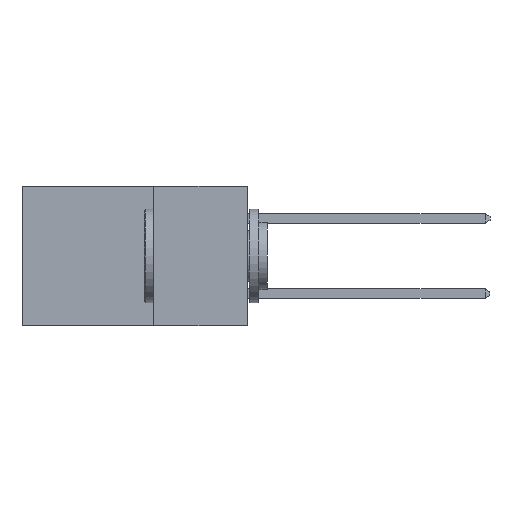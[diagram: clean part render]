
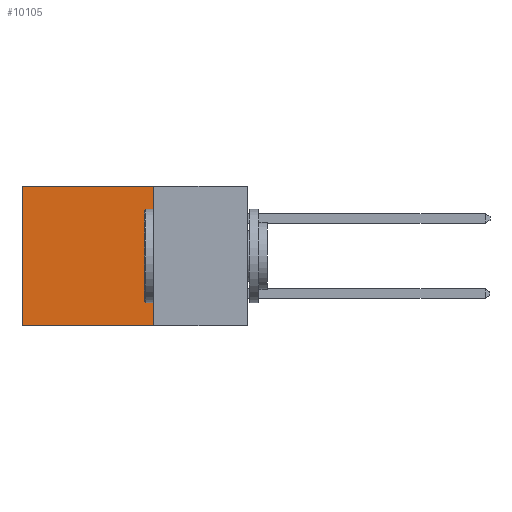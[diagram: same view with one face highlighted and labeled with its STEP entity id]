
A CAD part, left-side view. The second image highlights one B-rep face of the part: STEP entity #10105.
In plain terms, the highlighted planar face has unit normal (-1, 0, 0).
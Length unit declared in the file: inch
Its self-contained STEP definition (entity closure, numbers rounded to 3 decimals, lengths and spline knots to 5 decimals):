
#610 = LINE ( 'NONE', #11379, #5874 ) ;
#1391 = CARTESIAN_POINT ( 'NONE',  ( 0.298, 0.25, 0. ) ) ;
#1639 = LINE ( 'NONE', #3011, #11929 ) ;
#1975 = ORIENTED_EDGE ( 'NONE', *, *, #4548, .T. ) ;
#2060 = DIRECTION ( 'NONE',  ( 0., 0., -1. ) ) ;
#2175 = VERTEX_POINT ( 'NONE', #12620 ) ;
#2639 = CARTESIAN_POINT ( 'NONE',  ( 0.298, 0.25, 0. ) ) ;
#3011 = CARTESIAN_POINT ( 'NONE',  ( 0.298, 0.25, -0.37 ) ) ;
#3275 = EDGE_CURVE ( 'NONE', #7456, #2175, #12060, .T. ) ;
#4349 = CARTESIAN_POINT ( 'NONE',  ( 0.298, 0.25, 0. ) ) ;
#4428 = ORIENTED_EDGE ( 'NONE', *, *, #9059, .T. ) ;
#4548 = EDGE_CURVE ( 'NONE', #10939, #9738, #610, .T. ) ;
#4554 = DIRECTION ( 'NONE',  ( 1., 0., 0. ) ) ;
#5874 = VECTOR ( 'NONE', #9439, 39.37008 ) ;
#5966 = CARTESIAN_POINT ( 'NONE',  ( 0.298, 0.6, 0. ) ) ;
#6761 = VECTOR ( 'NONE', #2060, 39.37008 ) ;
#6915 = CARTESIAN_POINT ( 'NONE',  ( 0.298, 0.6, -0.37 ) ) ;
#6954 = VECTOR ( 'NONE', #10954, 39.37008 ) ;
#7062 = ORIENTED_EDGE ( 'NONE', *, *, #3275, .F. ) ;
#7456 = VERTEX_POINT ( 'NONE', #4349 ) ;
#7771 = FACE_OUTER_BOUND ( 'NONE', #8663, .T. ) ;
#8602 = ORIENTED_EDGE ( 'NONE', *, *, #12000, .F. ) ;
#8663 = EDGE_LOOP ( 'NONE', ( #1975, #8602, #7062, #4428 ) ) ;
#9059 = EDGE_CURVE ( 'NONE', #7456, #10939, #10034, .T. ) ;
#9439 = DIRECTION ( 'NONE',  ( 0., 0., -1. ) ) ;
#9738 = VERTEX_POINT ( 'NONE', #6915 ) ;
#9777 = CARTESIAN_POINT ( 'NONE',  ( 0.298, 0.25, 0. ) ) ;
#9826 = PLANE ( 'NONE',  #12117 ) ;
#10034 = LINE ( 'NONE', #2639, #6954 ) ;
#10105 = ADVANCED_FACE ( 'NONE', ( #7771 ), #9826, .F. ) ;
#10939 = VERTEX_POINT ( 'NONE', #5966 ) ;
#10954 = DIRECTION ( 'NONE',  ( 0., 1., 0. ) ) ;
#11379 = CARTESIAN_POINT ( 'NONE',  ( 0.298, 0.6, 0. ) ) ;
#11712 = DIRECTION ( 'NONE',  ( 0., 0., -1. ) ) ;
#11929 = VECTOR ( 'NONE', #13179, 39.37008 ) ;
#12000 = EDGE_CURVE ( 'NONE', #2175, #9738, #1639, .T. ) ;
#12060 = LINE ( 'NONE', #9777, #6761 ) ;
#12117 = AXIS2_PLACEMENT_3D ( 'NONE', #1391, #4554, #11712 ) ;
#12620 = CARTESIAN_POINT ( 'NONE',  ( 0.298, 0.25, -0.37 ) ) ;
#13179 = DIRECTION ( 'NONE',  ( 0., 1., 0. ) ) ;
